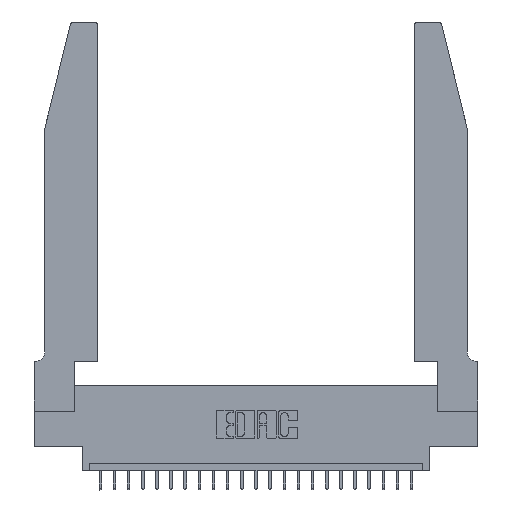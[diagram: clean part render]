
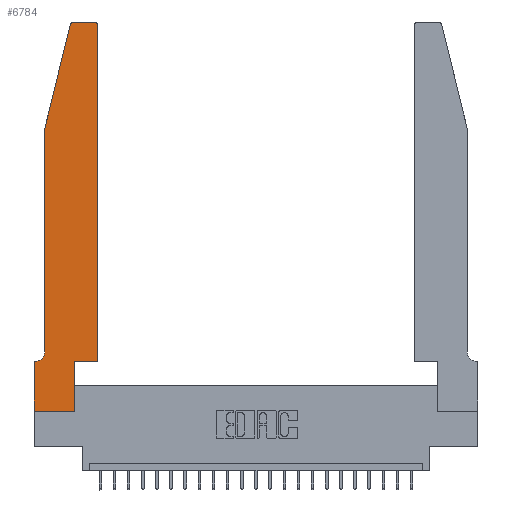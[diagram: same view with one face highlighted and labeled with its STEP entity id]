
A CAD part, top view. The second image highlights one B-rep face of the part: STEP entity #6784.
In plain terms, the highlighted planar face has unit normal (0, 0, 1).
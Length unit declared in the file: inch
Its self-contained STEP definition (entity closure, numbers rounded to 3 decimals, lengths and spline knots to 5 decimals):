
#25 = VERTEX_POINT ( 'NONE', #9488 ) ;
#865 = DIRECTION ( 'NONE',  ( 1., 0., 0. ) ) ;
#1053 = LINE ( 'NONE', #5899, #8126 ) ;
#1978 = CARTESIAN_POINT ( 'NONE',  ( 0.4205, 2.72, 0.37 ) ) ;
#2034 = ORIENTED_EDGE ( 'NONE', *, *, #12440, .T. ) ;
#2738 = ORIENTED_EDGE ( 'NONE', *, *, #13035, .T. ) ;
#3490 = CARTESIAN_POINT ( 'NONE',  ( 0.2605, 2.75, 0.37 ) ) ;
#3492 = DIRECTION ( 'NONE',  ( 0., -1., 0. ) ) ;
#3610 = EDGE_CURVE ( 'NONE', #7276, #24275, #8332, .T. ) ;
#4107 = EDGE_CURVE ( 'NONE', #16067, #9297, #21499, .T. ) ;
#4293 = ORIENTED_EDGE ( 'NONE', *, *, #4107, .T. ) ;
#4514 = CARTESIAN_POINT ( 'NONE',  ( 0.284, 2.72, 0.37 ) ) ;
#4601 = DIRECTION ( 'NONE',  ( 0., 1., 0. ) ) ;
#5119 = CIRCLE ( 'NONE', #24002, 0.03 ) ;
#5505 = DIRECTION ( 'NONE',  ( 0., 1., 0. ) ) ;
#5628 = AXIS2_PLACEMENT_3D ( 'NONE', #16740, #12473, #12981 ) ;
#5636 = DIRECTION ( 'NONE',  ( -1., 0., 0. ) ) ;
#5899 = CARTESIAN_POINT ( 'NONE',  ( 0.4505, 0.35, 0.37 ) ) ;
#6011 = VECTOR ( 'NONE', #5636, 39.37008 ) ;
#6204 = VERTEX_POINT ( 'NONE', #18156 ) ;
#6322 = EDGE_CURVE ( 'NONE', #19001, #9503, #18780, .T. ) ;
#6449 = VERTEX_POINT ( 'NONE', #11237 ) ;
#6452 = CARTESIAN_POINT ( 'NONE',  ( 0.4505, 0.35, 0.37 ) ) ;
#6485 = EDGE_LOOP ( 'NONE', ( #12828, #2034, #22823, #16706, #2738, #20289, #8852, #9352, #15494, #14995, #4293, #21486 ) ) ;
#6534 = CARTESIAN_POINT ( 'NONE',  ( 0., 0., 0.37 ) ) ;
#6784 = ADVANCED_FACE ( 'NONE', ( #24400 ), #18629, .T. ) ;
#7243 = EDGE_CURVE ( 'NONE', #9782, #6449, #15201, .T. ) ;
#7276 = VERTEX_POINT ( 'NONE', #7391 ) ;
#7292 = EDGE_CURVE ( 'NONE', #24275, #15255, #22735, .T. ) ;
#7391 = CARTESIAN_POINT ( 'NONE',  ( 0., 0., 0.37 ) ) ;
#7509 = DIRECTION ( 'NONE',  ( 0., 0., 1. ) ) ;
#7639 = DIRECTION ( 'NONE',  ( 1., 0., 0. ) ) ;
#8126 = VECTOR ( 'NONE', #9806, 39.37008 ) ;
#8332 = LINE ( 'NONE', #16003, #24231 ) ;
#8363 = CARTESIAN_POINT ( 'NONE',  ( 0.25487, 2.72718, 0.37 ) ) ;
#8463 = VECTOR ( 'NONE', #5505, 39.37008 ) ;
#8852 = ORIENTED_EDGE ( 'NONE', *, *, #19348, .T. ) ;
#9297 = VERTEX_POINT ( 'NONE', #16182 ) ;
#9352 = ORIENTED_EDGE ( 'NONE', *, *, #3610, .T. ) ;
#9488 = CARTESIAN_POINT ( 'NONE',  ( 0.284, 2.75, 0.37 ) ) ;
#9503 = VERTEX_POINT ( 'NONE', #20945 ) ;
#9782 = VERTEX_POINT ( 'NONE', #8363 ) ;
#9806 = DIRECTION ( 'NONE',  ( 1., 0., 0. ) ) ;
#10053 = CARTESIAN_POINT ( 'NONE',  ( 0.2865, 0.35, 0.37 ) ) ;
#10579 = LINE ( 'NONE', #11311, #18916 ) ;
#11237 = CARTESIAN_POINT ( 'NONE',  ( 0.0755, 2., 0.37 ) ) ;
#11311 = CARTESIAN_POINT ( 'NONE',  ( 0.0755, 2., 0.37 ) ) ;
#11645 = VECTOR ( 'NONE', #24616, 39.37008 ) ;
#12428 = CARTESIAN_POINT ( 'NONE',  ( 0.4505, 0.35, 0.37 ) ) ;
#12440 = EDGE_CURVE ( 'NONE', #25, #9782, #5119, .T. ) ;
#12473 = DIRECTION ( 'NONE',  ( 0., 0., 1. ) ) ;
#12828 = ORIENTED_EDGE ( 'NONE', *, *, #16383, .T. ) ;
#12981 = DIRECTION ( 'NONE',  ( 1., 0., 0. ) ) ;
#13035 = EDGE_CURVE ( 'NONE', #6204, #19001, #24418, .T. ) ;
#13767 = DIRECTION ( 'NONE',  ( 0., 0., -1. ) ) ;
#13947 = CIRCLE ( 'NONE', #19162, 0.03 ) ;
#14995 = ORIENTED_EDGE ( 'NONE', *, *, #19650, .T. ) ;
#15201 = LINE ( 'NONE', #17082, #11645 ) ;
#15255 = VERTEX_POINT ( 'NONE', #10053 ) ;
#15444 = VECTOR ( 'NONE', #4601, 39.37008 ) ;
#15494 = ORIENTED_EDGE ( 'NONE', *, *, #7292, .T. ) ;
#15527 = CARTESIAN_POINT ( 'NONE',  ( 0.0055, 0.42, 0.37 ) ) ;
#15647 = VERTEX_POINT ( 'NONE', #17812 ) ;
#15977 = DIRECTION ( 'NONE',  ( 0., 0., 1. ) ) ;
#16003 = CARTESIAN_POINT ( 'NONE',  ( 0., 0., 0.37 ) ) ;
#16067 = VERTEX_POINT ( 'NONE', #6452 ) ;
#16182 = CARTESIAN_POINT ( 'NONE',  ( 0.4505, 2.72, 0.37 ) ) ;
#16383 = EDGE_CURVE ( 'NONE', #15647, #25, #24374, .T. ) ;
#16625 = CARTESIAN_POINT ( 'NONE',  ( 0.0055, 0.35, 0.37 ) ) ;
#16706 = ORIENTED_EDGE ( 'NONE', *, *, #17710, .T. ) ;
#16740 = CARTESIAN_POINT ( 'NONE',  ( 0., 0.35, 0.37 ) ) ;
#16959 = CARTESIAN_POINT ( 'NONE',  ( 0.2865, 0.35, 0.37 ) ) ;
#17082 = CARTESIAN_POINT ( 'NONE',  ( 0.0755, 2., 0.37 ) ) ;
#17202 = AXIS2_PLACEMENT_3D ( 'NONE', #15527, #13767, #23057 ) ;
#17710 = EDGE_CURVE ( 'NONE', #6449, #6204, #10579, .T. ) ;
#17812 = CARTESIAN_POINT ( 'NONE',  ( 0.4205, 2.75, 0.37 ) ) ;
#18156 = CARTESIAN_POINT ( 'NONE',  ( 0.0755, 0.42, 0.37 ) ) ;
#18278 = DIRECTION ( 'NONE',  ( -1., 0., 0. ) ) ;
#18629 = PLANE ( 'NONE',  #5628 ) ;
#18780 = LINE ( 'NONE', #20664, #20459 ) ;
#18916 = VECTOR ( 'NONE', #3492, 39.37008 ) ;
#19001 = VERTEX_POINT ( 'NONE', #16625 ) ;
#19162 = AXIS2_PLACEMENT_3D ( 'NONE', #1978, #7509, #7639 ) ;
#19348 = EDGE_CURVE ( 'NONE', #9503, #7276, #23761, .T. ) ;
#19650 = EDGE_CURVE ( 'NONE', #15255, #16067, #1053, .T. ) ;
#19766 = VECTOR ( 'NONE', #22001, 39.37008 ) ;
#20289 = ORIENTED_EDGE ( 'NONE', *, *, #6322, .T. ) ;
#20459 = VECTOR ( 'NONE', #18278, 39.37008 ) ;
#20664 = CARTESIAN_POINT ( 'NONE',  ( 0.0755, 0.35, 0.37 ) ) ;
#20935 = CARTESIAN_POINT ( 'NONE',  ( 0.2865, 0., 0.37 ) ) ;
#20945 = CARTESIAN_POINT ( 'NONE',  ( 0., 0.35, 0.37 ) ) ;
#21486 = ORIENTED_EDGE ( 'NONE', *, *, #24566, .T. ) ;
#21499 = LINE ( 'NONE', #12428, #15444 ) ;
#22001 = DIRECTION ( 'NONE',  ( 0., -1., 0. ) ) ;
#22735 = LINE ( 'NONE', #16959, #8463 ) ;
#22823 = ORIENTED_EDGE ( 'NONE', *, *, #7243, .T. ) ;
#23057 = DIRECTION ( 'NONE',  ( -1., 0., 0. ) ) ;
#23418 = DIRECTION ( 'NONE',  ( 1., 0., 0. ) ) ;
#23761 = LINE ( 'NONE', #6534, #19766 ) ;
#24002 = AXIS2_PLACEMENT_3D ( 'NONE', #4514, #15977, #865 ) ;
#24231 = VECTOR ( 'NONE', #23418, 39.37008 ) ;
#24275 = VERTEX_POINT ( 'NONE', #20935 ) ;
#24374 = LINE ( 'NONE', #3490, #6011 ) ;
#24400 = FACE_OUTER_BOUND ( 'NONE', #6485, .T. ) ;
#24418 = CIRCLE ( 'NONE', #17202, 0.07 ) ;
#24566 = EDGE_CURVE ( 'NONE', #9297, #15647, #13947, .T. ) ;
#24616 = DIRECTION ( 'NONE',  ( -0.239, -0.971, 0. ) ) ;
